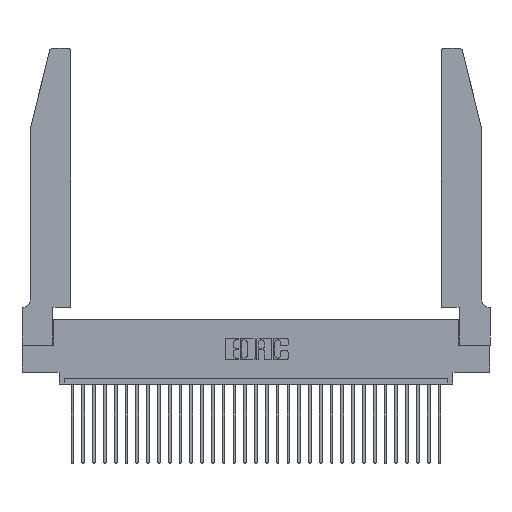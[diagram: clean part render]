
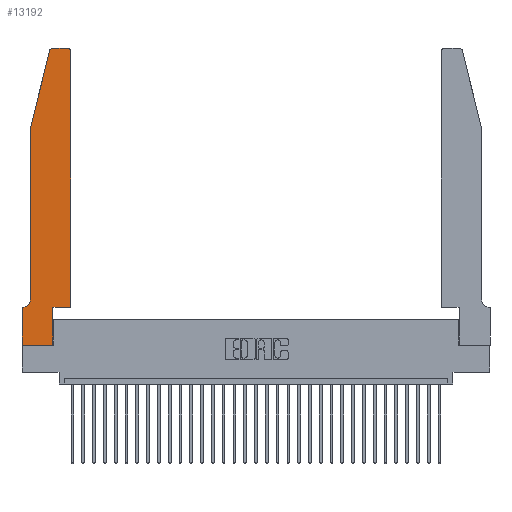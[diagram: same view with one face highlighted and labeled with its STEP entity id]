
A CAD part, top view. The second image highlights one B-rep face of the part: STEP entity #13192.
In plain terms, the highlighted planar face has unit normal (0, 0, 1).
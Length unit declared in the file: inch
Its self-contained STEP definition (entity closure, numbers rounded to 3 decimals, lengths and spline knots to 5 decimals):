
#251 = CARTESIAN_POINT ( 'NONE',  ( 0.2605, 2.75, 0.37 ) ) ;
#1607 = ORIENTED_EDGE ( 'NONE', *, *, #16330, .T. ) ;
#1995 = ORIENTED_EDGE ( 'NONE', *, *, #6449, .T. ) ;
#2192 = VERTEX_POINT ( 'NONE', #6421 ) ;
#2839 = VERTEX_POINT ( 'NONE', #9123 ) ;
#2858 = ORIENTED_EDGE ( 'NONE', *, *, #24013, .T. ) ;
#3005 = EDGE_CURVE ( 'NONE', #4330, #2192, #23105, .T. ) ;
#3162 = VERTEX_POINT ( 'NONE', #10251 ) ;
#3502 = CARTESIAN_POINT ( 'NONE',  ( 0.4505, 2.72, 0.37 ) ) ;
#4330 = VERTEX_POINT ( 'NONE', #9719 ) ;
#4937 = VERTEX_POINT ( 'NONE', #28014 ) ;
#4973 = VECTOR ( 'NONE', #28958, 39.37008 ) ;
#5214 = VERTEX_POINT ( 'NONE', #27356 ) ;
#5575 = EDGE_CURVE ( 'NONE', #16093, #4937, #11281, .T. ) ;
#5599 = CARTESIAN_POINT ( 'NONE',  ( 0., 0.35, 0.37 ) ) ;
#6421 = CARTESIAN_POINT ( 'NONE',  ( 0.25487, 2.72718, 0.37 ) ) ;
#6449 = EDGE_CURVE ( 'NONE', #15065, #12718, #15105, .T. ) ;
#6629 = VERTEX_POINT ( 'NONE', #30514 ) ;
#7060 = CARTESIAN_POINT ( 'NONE',  ( 0.4205, 2.72, 0.37 ) ) ;
#7694 = CARTESIAN_POINT ( 'NONE',  ( 0.4505, 0.35, 0.37 ) ) ;
#7836 = LINE ( 'NONE', #19118, #11742 ) ;
#8959 = EDGE_CURVE ( 'NONE', #26828, #5214, #22432, .T. ) ;
#8989 = VECTOR ( 'NONE', #10890, 39.37008 ) ;
#9009 = VERTEX_POINT ( 'NONE', #10272 ) ;
#9123 = CARTESIAN_POINT ( 'NONE',  ( 0.0755, 0.42, 0.37 ) ) ;
#9299 = EDGE_CURVE ( 'NONE', #4937, #4330, #19264, .T. ) ;
#9407 = DIRECTION ( 'NONE',  ( -1., 0., 0. ) ) ;
#9719 = CARTESIAN_POINT ( 'NONE',  ( 0.284, 2.75, 0.37 ) ) ;
#9991 = CARTESIAN_POINT ( 'NONE',  ( 0.0755, 2., 0.37 ) ) ;
#10244 = DIRECTION ( 'NONE',  ( -1., 0., 0. ) ) ;
#10251 = CARTESIAN_POINT ( 'NONE',  ( 0., 0., 0.37 ) ) ;
#10272 = CARTESIAN_POINT ( 'NONE',  ( 0.2865, 0., 0.37 ) ) ;
#10441 = LINE ( 'NONE', #7694, #29504 ) ;
#10746 = VECTOR ( 'NONE', #10244, 39.37008 ) ;
#10890 = DIRECTION ( 'NONE',  ( -0.239, -0.971, 0. ) ) ;
#11214 = CARTESIAN_POINT ( 'NONE',  ( 0., 0., 0.37 ) ) ;
#11281 = CIRCLE ( 'NONE', #27892, 0.03 ) ;
#11658 = ORIENTED_EDGE ( 'NONE', *, *, #28172, .T. ) ;
#11742 = VECTOR ( 'NONE', #11769, 39.37008 ) ;
#11769 = DIRECTION ( 'NONE',  ( 0., 1., 0. ) ) ;
#12718 = VERTEX_POINT ( 'NONE', #5599 ) ;
#12931 = DIRECTION ( 'NONE',  ( 0., -1., 0. ) ) ;
#12933 = DIRECTION ( 'NONE',  ( 0., 0., 1. ) ) ;
#13192 = ADVANCED_FACE ( 'NONE', ( #14795 ), #28095, .T. ) ;
#13537 = DIRECTION ( 'NONE',  ( 0., 1., 0. ) ) ;
#13717 = CARTESIAN_POINT ( 'NONE',  ( 0.0755, 2., 0.37 ) ) ;
#14165 = AXIS2_PLACEMENT_3D ( 'NONE', #21244, #18872, #23867 ) ;
#14556 = DIRECTION ( 'NONE',  ( 1., 0., 0. ) ) ;
#14735 = VECTOR ( 'NONE', #9407, 39.37008 ) ;
#14795 = FACE_OUTER_BOUND ( 'NONE', #24885, .T. ) ;
#14874 = EDGE_CURVE ( 'NONE', #12718, #3162, #24771, .T. ) ;
#14901 = LINE ( 'NONE', #9991, #28869 ) ;
#15061 = VECTOR ( 'NONE', #22638, 39.37008 ) ;
#15065 = VERTEX_POINT ( 'NONE', #30951 ) ;
#15105 = LINE ( 'NONE', #29180, #14735 ) ;
#15521 = LINE ( 'NONE', #11214, #24829 ) ;
#15529 = DIRECTION ( 'NONE',  ( 1., 0., 0. ) ) ;
#16093 = VERTEX_POINT ( 'NONE', #3502 ) ;
#16330 = EDGE_CURVE ( 'NONE', #3162, #9009, #15521, .T. ) ;
#16684 = EDGE_CURVE ( 'NONE', #5214, #16093, #10441, .T. ) ;
#17481 = ORIENTED_EDGE ( 'NONE', *, *, #31869, .T. ) ;
#18872 = DIRECTION ( 'NONE',  ( 0., 0., -1. ) ) ;
#19118 = CARTESIAN_POINT ( 'NONE',  ( 0.2865, 0.35, 0.37 ) ) ;
#19264 = LINE ( 'NONE', #251, #10746 ) ;
#20266 = CARTESIAN_POINT ( 'NONE',  ( 0., 0.35, 0.37 ) ) ;
#20534 = AXIS2_PLACEMENT_3D ( 'NONE', #24523, #27240, #14556 ) ;
#20698 = ORIENTED_EDGE ( 'NONE', *, *, #3005, .T. ) ;
#21244 = CARTESIAN_POINT ( 'NONE',  ( 0.0055, 0.42, 0.37 ) ) ;
#21324 = EDGE_CURVE ( 'NONE', #9009, #26828, #7836, .T. ) ;
#22432 = LINE ( 'NONE', #27536, #15061 ) ;
#22638 = DIRECTION ( 'NONE',  ( 1., 0., 0. ) ) ;
#23077 = DIRECTION ( 'NONE',  ( 1., 0., 0. ) ) ;
#23105 = CIRCLE ( 'NONE', #20534, 0.03 ) ;
#23683 = ORIENTED_EDGE ( 'NONE', *, *, #16684, .T. ) ;
#23686 = DIRECTION ( 'NONE',  ( 1., 0., 0. ) ) ;
#23867 = DIRECTION ( 'NONE',  ( -1., 0., 0. ) ) ;
#24013 = EDGE_CURVE ( 'NONE', #6629, #2839, #14901, .T. ) ;
#24305 = CIRCLE ( 'NONE', #14165, 0.07 ) ;
#24523 = CARTESIAN_POINT ( 'NONE',  ( 0.284, 2.72, 0.37 ) ) ;
#24557 = ORIENTED_EDGE ( 'NONE', *, *, #9299, .T. ) ;
#24771 = LINE ( 'NONE', #30700, #4973 ) ;
#24829 = VECTOR ( 'NONE', #23686, 39.37008 ) ;
#24885 = EDGE_LOOP ( 'NONE', ( #24557, #20698, #11658, #2858, #17481, #1995, #30173, #1607, #29211, #27667, #23683, #26708 ) ) ;
#25484 = DIRECTION ( 'NONE',  ( 0., 0., 1. ) ) ;
#26708 = ORIENTED_EDGE ( 'NONE', *, *, #5575, .T. ) ;
#26828 = VERTEX_POINT ( 'NONE', #30318 ) ;
#27240 = DIRECTION ( 'NONE',  ( 0., 0., 1. ) ) ;
#27356 = CARTESIAN_POINT ( 'NONE',  ( 0.4505, 0.35, 0.37 ) ) ;
#27536 = CARTESIAN_POINT ( 'NONE',  ( 0.4505, 0.35, 0.37 ) ) ;
#27667 = ORIENTED_EDGE ( 'NONE', *, *, #8959, .T. ) ;
#27892 = AXIS2_PLACEMENT_3D ( 'NONE', #7060, #25484, #23077 ) ;
#28014 = CARTESIAN_POINT ( 'NONE',  ( 0.4205, 2.75, 0.37 ) ) ;
#28095 = PLANE ( 'NONE',  #30344 ) ;
#28172 = EDGE_CURVE ( 'NONE', #2192, #6629, #30379, .T. ) ;
#28869 = VECTOR ( 'NONE', #12931, 39.37008 ) ;
#28958 = DIRECTION ( 'NONE',  ( 0., -1., 0. ) ) ;
#29180 = CARTESIAN_POINT ( 'NONE',  ( 0.0755, 0.35, 0.37 ) ) ;
#29211 = ORIENTED_EDGE ( 'NONE', *, *, #21324, .T. ) ;
#29504 = VECTOR ( 'NONE', #13537, 39.37008 ) ;
#30173 = ORIENTED_EDGE ( 'NONE', *, *, #14874, .T. ) ;
#30318 = CARTESIAN_POINT ( 'NONE',  ( 0.2865, 0.35, 0.37 ) ) ;
#30344 = AXIS2_PLACEMENT_3D ( 'NONE', #20266, #12933, #15529 ) ;
#30379 = LINE ( 'NONE', #13717, #8989 ) ;
#30514 = CARTESIAN_POINT ( 'NONE',  ( 0.0755, 2., 0.37 ) ) ;
#30700 = CARTESIAN_POINT ( 'NONE',  ( 0., 0., 0.37 ) ) ;
#30951 = CARTESIAN_POINT ( 'NONE',  ( 0.0055, 0.35, 0.37 ) ) ;
#31869 = EDGE_CURVE ( 'NONE', #2839, #15065, #24305, .T. ) ;
